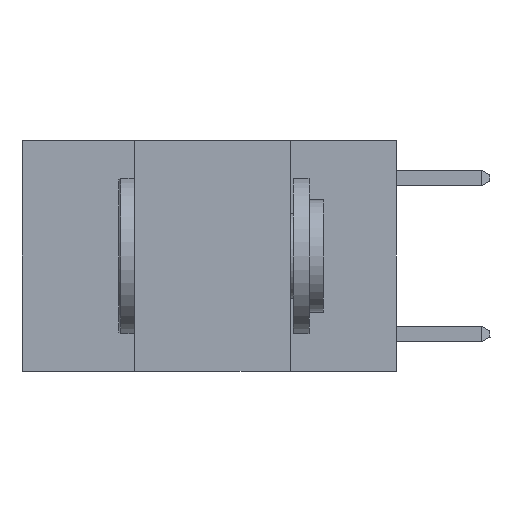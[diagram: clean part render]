
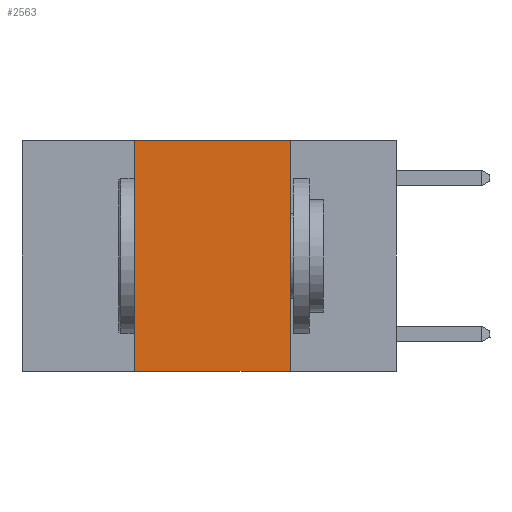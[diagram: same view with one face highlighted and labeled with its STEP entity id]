
A CAD part, left-side view. The second image highlights one B-rep face of the part: STEP entity #2563.
In plain terms, the highlighted planar face has unit normal (-1, 0, 0).
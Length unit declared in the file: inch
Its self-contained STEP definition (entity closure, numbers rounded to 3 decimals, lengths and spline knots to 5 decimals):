
#190 = VECTOR ( 'NONE', #16708, 39.37008 ) ;
#664 = CARTESIAN_POINT ( 'NONE',  ( 0., 0.42, 0. ) ) ;
#807 = CARTESIAN_POINT ( 'NONE',  ( 0., 0.17, -0.37 ) ) ;
#1082 = VECTOR ( 'NONE', #16094, 39.37008 ) ;
#1797 = VERTEX_POINT ( 'NONE', #807 ) ;
#1881 = CARTESIAN_POINT ( 'NONE',  ( 0., 0.42, -0.37 ) ) ;
#2503 = PLANE ( 'NONE',  #14466 ) ;
#2563 = ADVANCED_FACE ( 'NONE', ( #16672 ), #2503, .F. ) ;
#3019 = EDGE_CURVE ( 'NONE', #15600, #19151, #12534, .T. ) ;
#3318 = EDGE_LOOP ( 'NONE', ( #7875, #15945, #16426, #8355 ) ) ;
#5334 = LINE ( 'NONE', #5485, #1082 ) ;
#5485 = CARTESIAN_POINT ( 'NONE',  ( 0., 0.6, -0.37 ) ) ;
#5603 = VECTOR ( 'NONE', #18192, 39.37008 ) ;
#5645 = DIRECTION ( 'NONE',  ( 1., 0., 0. ) ) ;
#6083 = LINE ( 'NONE', #13618, #5603 ) ;
#6187 = EDGE_CURVE ( 'NONE', #15471, #15600, #6795, .T. ) ;
#6795 = LINE ( 'NONE', #664, #10341 ) ;
#7875 = ORIENTED_EDGE ( 'NONE', *, *, #14061, .F. ) ;
#8355 = ORIENTED_EDGE ( 'NONE', *, *, #14885, .T. ) ;
#10146 = CARTESIAN_POINT ( 'NONE',  ( 0., 0.6, 0. ) ) ;
#10341 = VECTOR ( 'NONE', #13018, 39.37008 ) ;
#12534 = LINE ( 'NONE', #15161, #190 ) ;
#13018 = DIRECTION ( 'NONE',  ( 0., 0., 1. ) ) ;
#13618 = CARTESIAN_POINT ( 'NONE',  ( 0., 0.17, 0. ) ) ;
#14061 = EDGE_CURVE ( 'NONE', #19151, #1797, #6083, .T. ) ;
#14387 = CARTESIAN_POINT ( 'NONE',  ( 0., 0.42, 0. ) ) ;
#14466 = AXIS2_PLACEMENT_3D ( 'NONE', #10146, #5645, #16254 ) ;
#14885 = EDGE_CURVE ( 'NONE', #15471, #1797, #5334, .T. ) ;
#15161 = CARTESIAN_POINT ( 'NONE',  ( 0., 0.6, 0. ) ) ;
#15471 = VERTEX_POINT ( 'NONE', #1881 ) ;
#15600 = VERTEX_POINT ( 'NONE', #14387 ) ;
#15945 = ORIENTED_EDGE ( 'NONE', *, *, #3019, .F. ) ;
#16094 = DIRECTION ( 'NONE',  ( 0., -1., 0. ) ) ;
#16254 = DIRECTION ( 'NONE',  ( 0., 0., -1. ) ) ;
#16426 = ORIENTED_EDGE ( 'NONE', *, *, #6187, .F. ) ;
#16672 = FACE_OUTER_BOUND ( 'NONE', #3318, .T. ) ;
#16708 = DIRECTION ( 'NONE',  ( 0., -1., 0. ) ) ;
#16730 = CARTESIAN_POINT ( 'NONE',  ( 0., 0.17, 0. ) ) ;
#18192 = DIRECTION ( 'NONE',  ( 0., 0., -1. ) ) ;
#19151 = VERTEX_POINT ( 'NONE', #16730 ) ;
